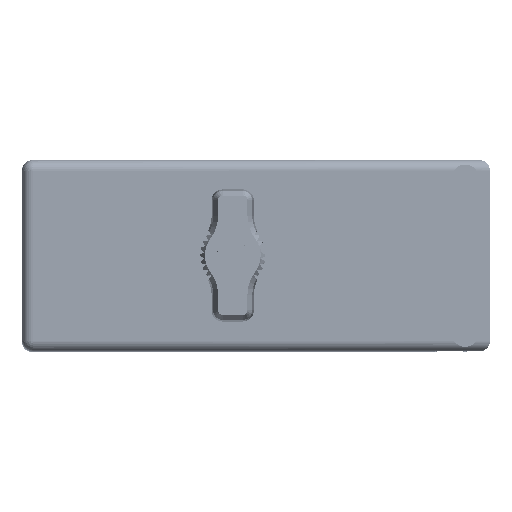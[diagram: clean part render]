
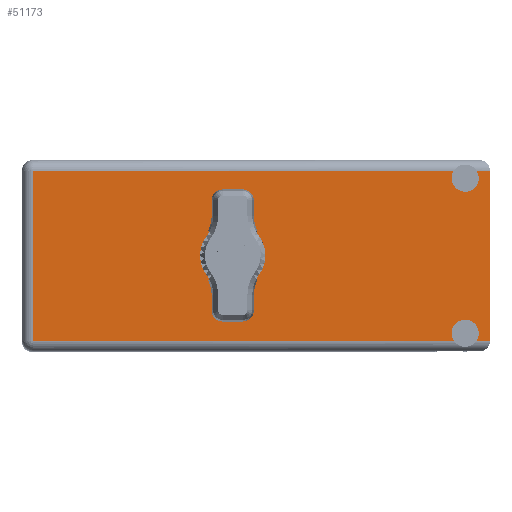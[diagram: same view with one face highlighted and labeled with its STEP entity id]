
A CAD part, top view. The second image highlights one B-rep face of the part: STEP entity #51173.
In plain terms, the highlighted face is planar.
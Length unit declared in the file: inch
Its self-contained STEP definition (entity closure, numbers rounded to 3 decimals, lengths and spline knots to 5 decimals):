
#2070 = CARTESIAN_POINT ( 'NONE',  ( 1.359, 1.775, -0.617 ) ) ;
#4090 = EDGE_CURVE ( 'NONE', #47837, #98412, #33954, .T. ) ;
#5221 = CARTESIAN_POINT ( 'NONE',  ( 2.858, 1.775, -0.2045 ) ) ;
#5426 = VERTEX_POINT ( 'NONE', #43285 ) ;
#6773 = AXIS2_PLACEMENT_3D ( 'NONE', #15592, #38260, #76579 ) ;
#7054 = FACE_BOUND ( 'NONE', #93687, .T. ) ;
#8755 = CARTESIAN_POINT ( 'NONE',  ( 2.93181, 1.775, -1.164 ) ) ;
#9434 = CARTESIAN_POINT ( 'NONE',  ( 2.858, 1.775, -1.117 ) ) ;
#12588 = ORIENTED_EDGE ( 'NONE', *, *, #34912, .T. ) ;
#13079 = DIRECTION ( 'NONE',  ( 1., 0., 0. ) ) ;
#13455 = DIRECTION ( 'NONE',  ( 0., 1., 0. ) ) ;
#13659 = VECTOR ( 'NONE', #61882, 39.37008 ) ;
#14964 = LINE ( 'NONE', #29395, #33928 ) ;
#15592 = CARTESIAN_POINT ( 'NONE',  ( 2.858, 1.775, -1.117 ) ) ;
#15880 = CIRCLE ( 'NONE', #52115, 0.0875 ) ;
#16443 = ORIENTED_EDGE ( 'NONE', *, *, #4090, .T. ) ;
#17406 = DIRECTION ( 'NONE',  ( 0., 0., 1. ) ) ;
#17848 = EDGE_CURVE ( 'NONE', #43865, #98412, #48321, .T. ) ;
#17996 = EDGE_CURVE ( 'NONE', #5426, #97344, #14964, .T. ) ;
#18197 = CIRCLE ( 'NONE', #50627, 0.0875 ) ;
#18422 = CARTESIAN_POINT ( 'NONE',  ( 2.858, 1.775, -0.117 ) ) ;
#19492 = EDGE_CURVE ( 'NONE', #75846, #32179, #94149, .T. ) ;
#19535 = ORIENTED_EDGE ( 'NONE', *, *, #84118, .F. ) ;
#21042 = DIRECTION ( 'NONE',  ( 0., 0., 1. ) ) ;
#21275 = ORIENTED_EDGE ( 'NONE', *, *, #48081, .T. ) ;
#22460 = ORIENTED_EDGE ( 'NONE', *, *, #46334, .F. ) ;
#22521 = ORIENTED_EDGE ( 'NONE', *, *, #28126, .F. ) ;
#22715 = LINE ( 'NONE', #51134, #91894 ) ;
#25559 = CARTESIAN_POINT ( 'NONE',  ( 3.018, 1.775, -1.164 ) ) ;
#26640 = CARTESIAN_POINT ( 'NONE',  ( 2.858, 1.775, -1.0295 ) ) ;
#27852 = VERTEX_POINT ( 'NONE', #42781 ) ;
#28126 = EDGE_CURVE ( 'NONE', #80587, #97344, #15880, .T. ) ;
#29088 = AXIS2_PLACEMENT_3D ( 'NONE', #90729, #98388, #52687 ) ;
#29395 = CARTESIAN_POINT ( 'NONE',  ( 3.018, 1.775, -0.07 ) ) ;
#32179 = VERTEX_POINT ( 'NONE', #87166 ) ;
#32652 = DIRECTION ( 'NONE',  ( 0., 0., 1. ) ) ;
#33928 = VECTOR ( 'NONE', #13079, 39.37008 ) ;
#33954 = LINE ( 'NONE', #52191, #13659 ) ;
#34379 = VECTOR ( 'NONE', #21042, 39.37008 ) ;
#34912 = EDGE_CURVE ( 'NONE', #50007, #5426, #73874, .T. ) ;
#38260 = DIRECTION ( 'NONE',  ( 0., 1., 0. ) ) ;
#39818 = DIRECTION ( 'NONE',  ( -1., 0., 0. ) ) ;
#42781 = CARTESIAN_POINT ( 'NONE',  ( 2.93181, 1.775, -0.07 ) ) ;
#43003 = CARTESIAN_POINT ( 'NONE',  ( 2.78419, 1.775, -0.07 ) ) ;
#43285 = CARTESIAN_POINT ( 'NONE',  ( 0.07, 1.775, -0.07 ) ) ;
#43824 = AXIS2_PLACEMENT_3D ( 'NONE', #98125, #13455, #59779 ) ;
#43865 = VERTEX_POINT ( 'NONE', #26640 ) ;
#43929 = LINE ( 'NONE', #98078, #34379 ) ;
#45378 = ORIENTED_EDGE ( 'NONE', *, *, #97627, .F. ) ;
#45819 = CARTESIAN_POINT ( 'NONE',  ( 3.018, 1.775, -0.07 ) ) ;
#46004 = CARTESIAN_POINT ( 'NONE',  ( 2.78419, 1.775, -1.164 ) ) ;
#46334 = EDGE_CURVE ( 'NONE', #27852, #80587, #18197, .T. ) ;
#46394 = DIRECTION ( 'NONE',  ( 0., 1., 0. ) ) ;
#47837 = VERTEX_POINT ( 'NONE', #25559 ) ;
#47952 = CIRCLE ( 'NONE', #6773, 0.0875 ) ;
#47999 = DIRECTION ( 'NONE',  ( 0., 1., 0. ) ) ;
#48026 = DIRECTION ( 'NONE',  ( 0., 0., 1. ) ) ;
#48081 = EDGE_CURVE ( 'NONE', #27852, #59988, #22715, .T. ) ;
#48321 = CIRCLE ( 'NONE', #63724, 0.0875 ) ;
#48877 = LINE ( 'NONE', #85498, #54828 ) ;
#50007 = VERTEX_POINT ( 'NONE', #83823 ) ;
#50627 = AXIS2_PLACEMENT_3D ( 'NONE', #18422, #95124, #88095 ) ;
#51134 = CARTESIAN_POINT ( 'NONE',  ( 3.018, 1.775, -0.07 ) ) ;
#51173 = ADVANCED_FACE ( 'NONE', ( #7054, #60700 ), #82741, .T. ) ;
#52115 = AXIS2_PLACEMENT_3D ( 'NONE', #89751, #46394, #48026 ) ;
#52191 = CARTESIAN_POINT ( 'NONE',  ( 0., 1.775, -1.164 ) ) ;
#52687 = DIRECTION ( 'NONE',  ( 0., 0., 1. ) ) ;
#54828 = VECTOR ( 'NONE', #39818, 39.37008 ) ;
#54857 = ORIENTED_EDGE ( 'NONE', *, *, #76883, .T. ) ;
#55401 = DIRECTION ( 'NONE',  ( 0., 1., 0. ) ) ;
#57888 = ORIENTED_EDGE ( 'NONE', *, *, #17848, .F. ) ;
#58525 = DIRECTION ( 'NONE',  ( 1., 0., 0. ) ) ;
#59779 = DIRECTION ( 'NONE',  ( 0., 0., 1. ) ) ;
#59988 = VERTEX_POINT ( 'NONE', #45819 ) ;
#60700 = FACE_OUTER_BOUND ( 'NONE', #69807, .T. ) ;
#61882 = DIRECTION ( 'NONE',  ( -1., 0., 0. ) ) ;
#63724 = AXIS2_PLACEMENT_3D ( 'NONE', #9434, #55401, #17406 ) ;
#69807 = EDGE_LOOP ( 'NONE', ( #98319, #22521, #22460, #21275, #19535, #16443, #57888, #45378, #54857, #12588 ) ) ;
#70656 = CARTESIAN_POINT ( 'NONE',  ( 0.07, 1.775, -1.234 ) ) ;
#73245 = ORIENTED_EDGE ( 'NONE', *, *, #19492, .F. ) ;
#73874 = LINE ( 'NONE', #70656, #90437 ) ;
#74763 = CARTESIAN_POINT ( 'NONE',  ( 1.359, 1.775, -0.742 ) ) ;
#75846 = VERTEX_POINT ( 'NONE', #74763 ) ;
#76579 = DIRECTION ( 'NONE',  ( 0., 0., 1. ) ) ;
#76883 = EDGE_CURVE ( 'NONE', #79596, #50007, #48877, .T. ) ;
#76969 = ORIENTED_EDGE ( 'NONE', *, *, #88421, .F. ) ;
#79596 = VERTEX_POINT ( 'NONE', #46004 ) ;
#80587 = VERTEX_POINT ( 'NONE', #5221 ) ;
#82741 = PLANE ( 'NONE',  #43824 ) ;
#83823 = CARTESIAN_POINT ( 'NONE',  ( 0.07, 1.775, -1.164 ) ) ;
#84118 = EDGE_CURVE ( 'NONE', #47837, #59988, #43929, .T. ) ;
#85498 = CARTESIAN_POINT ( 'NONE',  ( 0., 1.775, -1.164 ) ) ;
#87166 = CARTESIAN_POINT ( 'NONE',  ( 1.359, 1.775, -0.492 ) ) ;
#88095 = DIRECTION ( 'NONE',  ( 0., 0., 1. ) ) ;
#88421 = EDGE_CURVE ( 'NONE', #32179, #75846, #89611, .T. ) ;
#89611 = CIRCLE ( 'NONE', #29088, 0.125 ) ;
#89751 = CARTESIAN_POINT ( 'NONE',  ( 2.858, 1.775, -0.117 ) ) ;
#90437 = VECTOR ( 'NONE', #32652, 39.37008 ) ;
#90729 = CARTESIAN_POINT ( 'NONE',  ( 1.359, 1.775, -0.617 ) ) ;
#91894 = VECTOR ( 'NONE', #58525, 39.37008 ) ;
#93687 = EDGE_LOOP ( 'NONE', ( #76969, #73245 ) ) ;
#94020 = DIRECTION ( 'NONE',  ( 0., 0., 1. ) ) ;
#94149 = CIRCLE ( 'NONE', #96448, 0.125 ) ;
#95124 = DIRECTION ( 'NONE',  ( 0., 1., 0. ) ) ;
#96448 = AXIS2_PLACEMENT_3D ( 'NONE', #2070, #47999, #94020 ) ;
#97344 = VERTEX_POINT ( 'NONE', #43003 ) ;
#97627 = EDGE_CURVE ( 'NONE', #79596, #43865, #47952, .T. ) ;
#98078 = CARTESIAN_POINT ( 'NONE',  ( 3.018, 1.775, 0. ) ) ;
#98125 = CARTESIAN_POINT ( 'NONE',  ( 0., 1.775, -1.234 ) ) ;
#98319 = ORIENTED_EDGE ( 'NONE', *, *, #17996, .T. ) ;
#98388 = DIRECTION ( 'NONE',  ( 0., 1., 0. ) ) ;
#98412 = VERTEX_POINT ( 'NONE', #8755 ) ;
